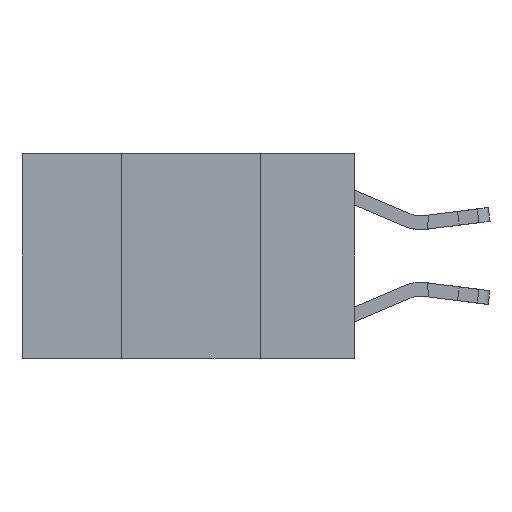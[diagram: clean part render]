
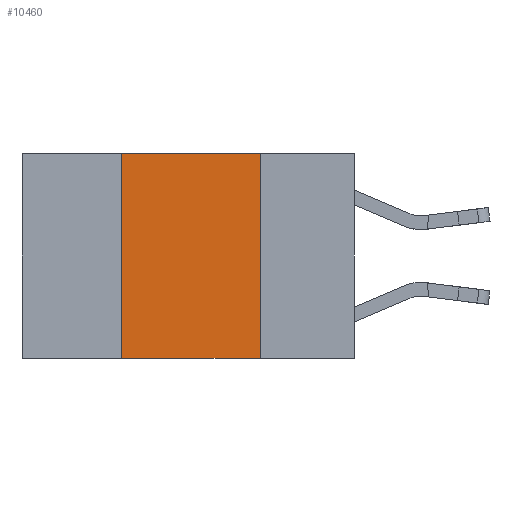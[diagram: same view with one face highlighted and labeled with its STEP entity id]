
A CAD part, left-side view. The second image highlights one B-rep face of the part: STEP entity #10460.
In plain terms, the highlighted planar face has unit normal (-1, 0, 0).
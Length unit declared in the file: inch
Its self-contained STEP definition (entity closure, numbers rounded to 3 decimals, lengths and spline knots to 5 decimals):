
#324 = DIRECTION ( 'NONE',  ( 0., -1., 0. ) ) ;
#753 = ORIENTED_EDGE ( 'NONE', *, *, #15722, .F. ) ;
#1725 = CARTESIAN_POINT ( 'NONE',  ( 0., 0.6, -0.37 ) ) ;
#1921 = CARTESIAN_POINT ( 'NONE',  ( 0., 0.6, 0. ) ) ;
#1981 = DIRECTION ( 'NONE',  ( 1., 0., 0. ) ) ;
#2015 = ORIENTED_EDGE ( 'NONE', *, *, #13661, .T. ) ;
#2613 = VERTEX_POINT ( 'NONE', #3396 ) ;
#2857 = DIRECTION ( 'NONE',  ( 0., 0., -1. ) ) ;
#3132 = EDGE_CURVE ( 'NONE', #8820, #2613, #16393, .T. ) ;
#3396 = CARTESIAN_POINT ( 'NONE',  ( 0., 0.17, 0. ) ) ;
#3569 = CARTESIAN_POINT ( 'NONE',  ( 0., 0.17, -0.37 ) ) ;
#4380 = EDGE_LOOP ( 'NONE', ( #753, #10380, #9922, #2015 ) ) ;
#5162 = DIRECTION ( 'NONE',  ( 0., 0., 1. ) ) ;
#5332 = VERTEX_POINT ( 'NONE', #10470 ) ;
#5869 = VECTOR ( 'NONE', #2857, 39.37008 ) ;
#5907 = VECTOR ( 'NONE', #324, 39.37008 ) ;
#7176 = LINE ( 'NONE', #9863, #5869 ) ;
#8820 = VERTEX_POINT ( 'NONE', #12164 ) ;
#9009 = FACE_OUTER_BOUND ( 'NONE', #4380, .T. ) ;
#9326 = CARTESIAN_POINT ( 'NONE',  ( 0., 0.42, 0. ) ) ;
#9577 = VECTOR ( 'NONE', #10177, 39.37008 ) ;
#9705 = VECTOR ( 'NONE', #5162, 39.37008 ) ;
#9863 = CARTESIAN_POINT ( 'NONE',  ( 0., 0.17, 0. ) ) ;
#9922 = ORIENTED_EDGE ( 'NONE', *, *, #17403, .F. ) ;
#10177 = DIRECTION ( 'NONE',  ( 0., -1., 0. ) ) ;
#10380 = ORIENTED_EDGE ( 'NONE', *, *, #3132, .F. ) ;
#10434 = PLANE ( 'NONE',  #12712 ) ;
#10460 = ADVANCED_FACE ( 'NONE', ( #9009 ), #10434, .F. ) ;
#10470 = CARTESIAN_POINT ( 'NONE',  ( 0., 0.42, -0.37 ) ) ;
#11791 = DIRECTION ( 'NONE',  ( 0., 0., -1. ) ) ;
#12164 = CARTESIAN_POINT ( 'NONE',  ( 0., 0.42, 0. ) ) ;
#12712 = AXIS2_PLACEMENT_3D ( 'NONE', #1921, #1981, #11791 ) ;
#13661 = EDGE_CURVE ( 'NONE', #5332, #14394, #16834, .T. ) ;
#14394 = VERTEX_POINT ( 'NONE', #3569 ) ;
#15722 = EDGE_CURVE ( 'NONE', #2613, #14394, #7176, .T. ) ;
#16393 = LINE ( 'NONE', #17010, #5907 ) ;
#16834 = LINE ( 'NONE', #1725, #9577 ) ;
#17010 = CARTESIAN_POINT ( 'NONE',  ( 0., 0.6, 0. ) ) ;
#17391 = LINE ( 'NONE', #9326, #9705 ) ;
#17403 = EDGE_CURVE ( 'NONE', #5332, #8820, #17391, .T. ) ;
